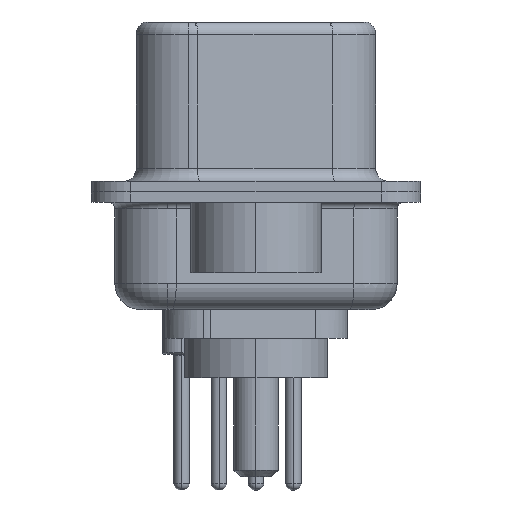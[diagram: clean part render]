
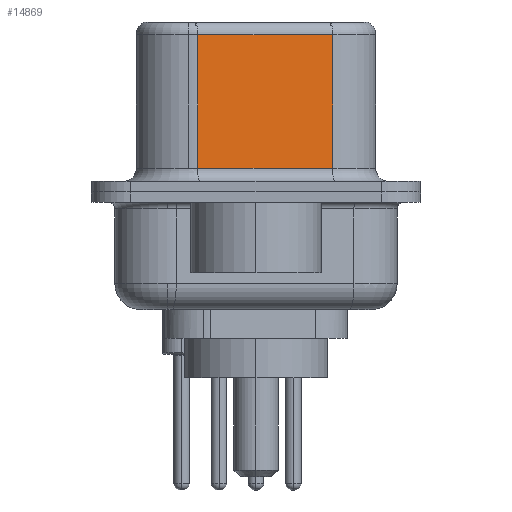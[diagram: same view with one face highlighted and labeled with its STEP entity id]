
A CAD part, left-side view. The second image highlights one B-rep face of the part: STEP entity #14869.
In plain terms, the highlighted planar face has unit normal (-0.985, -0.174, 0).
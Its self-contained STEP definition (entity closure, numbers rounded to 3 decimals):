
#2389 = CARTESIAN_POINT ( 'NONE',  ( 4.58, -2.927, 0.9 ) ) ;
#2501 = DIRECTION ( 'NONE',  ( -0.174, 0.985, 0. ) ) ;
#2695 = ORIENTED_EDGE ( 'NONE', *, *, #9993, .F. ) ;
#3297 = ORIENTED_EDGE ( 'NONE', *, *, #19951, .T. ) ;
#4294 = VECTOR ( 'NONE', #2501, 1000. ) ;
#4320 = CARTESIAN_POINT ( 'NONE',  ( 3.67, 2.233, 6.02 ) ) ;
#4688 = FACE_OUTER_BOUND ( 'NONE', #8938, .T. ) ;
#5393 = DIRECTION ( 'NONE',  ( 0.174, -0.985, 0. ) ) ;
#6088 = CARTESIAN_POINT ( 'NONE',  ( 4.58, -2.927, 0.9 ) ) ;
#6306 = VERTEX_POINT ( 'NONE', #6088 ) ;
#7194 = LINE ( 'NONE', #18796, #10843 ) ;
#7712 = DIRECTION ( 'NONE',  ( 0., 0., -1. ) ) ;
#7818 = CARTESIAN_POINT ( 'NONE',  ( 4.58, -2.927, 6.52 ) ) ;
#7827 = CARTESIAN_POINT ( 'NONE',  ( 4.58, -2.927, 6.52 ) ) ;
#8063 = VECTOR ( 'NONE', #5393, 1000. ) ;
#8532 = LINE ( 'NONE', #2389, #8063 ) ;
#8841 = LINE ( 'NONE', #14845, #4294 ) ;
#8938 = EDGE_LOOP ( 'NONE', ( #2695, #8940, #19802, #3297 ) ) ;
#8940 = ORIENTED_EDGE ( 'NONE', *, *, #12060, .T. ) ;
#9145 = DIRECTION ( 'NONE',  ( 0., 0., -1. ) ) ;
#9351 = DIRECTION ( 'NONE',  ( -0.174, 0.985, 0. ) ) ;
#9750 = AXIS2_PLACEMENT_3D ( 'NONE', #7818, #18906, #9351 ) ;
#9950 = VECTOR ( 'NONE', #9145, 1000. ) ;
#9993 = EDGE_CURVE ( 'NONE', #19178, #6306, #14104, .T. ) ;
#10017 = CARTESIAN_POINT ( 'NONE',  ( 4.58, -2.927, 6.02 ) ) ;
#10843 = VECTOR ( 'NONE', #7712, 1000. ) ;
#11036 = CARTESIAN_POINT ( 'NONE',  ( 3.67, 2.233, 0.9 ) ) ;
#12060 = EDGE_CURVE ( 'NONE', #19178, #13581, #8841, .T. ) ;
#13581 = VERTEX_POINT ( 'NONE', #4320 ) ;
#14104 = LINE ( 'NONE', #7827, #9950 ) ;
#14845 = CARTESIAN_POINT ( 'NONE',  ( 4.58, -2.927, 6.02 ) ) ;
#14869 = ADVANCED_FACE ( 'NONE', ( #4688 ), #17287, .F. ) ;
#17287 = PLANE ( 'NONE',  #9750 ) ;
#18434 = EDGE_CURVE ( 'NONE', #13581, #18486, #7194, .T. ) ;
#18486 = VERTEX_POINT ( 'NONE', #11036 ) ;
#18796 = CARTESIAN_POINT ( 'NONE',  ( 3.67, 2.233, 6.52 ) ) ;
#18906 = DIRECTION ( 'NONE',  ( 0.985, 0.174, 0. ) ) ;
#19178 = VERTEX_POINT ( 'NONE', #10017 ) ;
#19802 = ORIENTED_EDGE ( 'NONE', *, *, #18434, .T. ) ;
#19951 = EDGE_CURVE ( 'NONE', #18486, #6306, #8532, .T. ) ;
